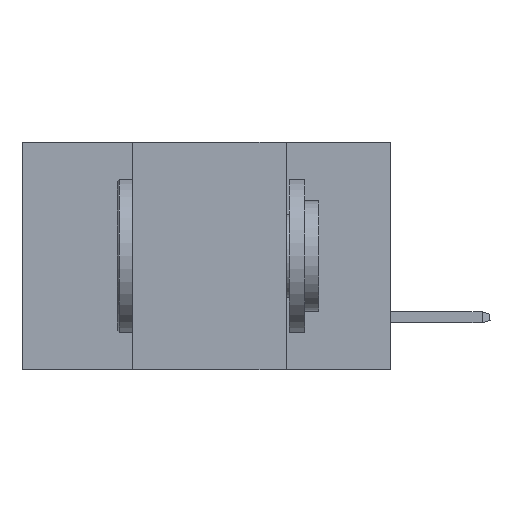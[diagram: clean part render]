
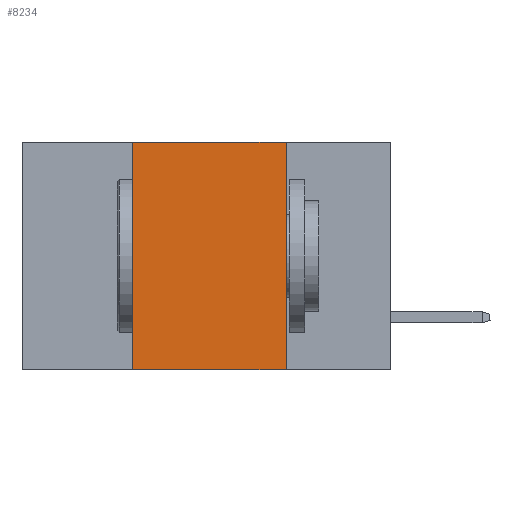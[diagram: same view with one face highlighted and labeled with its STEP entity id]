
A CAD part, left-side view. The second image highlights one B-rep face of the part: STEP entity #8234.
In plain terms, the highlighted planar face has unit normal (-1, 0, 0).
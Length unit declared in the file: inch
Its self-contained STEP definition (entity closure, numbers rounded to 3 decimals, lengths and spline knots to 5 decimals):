
#2219 = CARTESIAN_POINT ( 'NONE',  ( 0., 0.42, 0. ) ) ;
#3215 = ORIENTED_EDGE ( 'NONE', *, *, #3407, .F. ) ;
#3407 = EDGE_CURVE ( 'NONE', #5116, #25669, #23137, .T. ) ;
#4505 = EDGE_CURVE ( 'NONE', #23693, #37012, #13650, .T. ) ;
#5116 = VERTEX_POINT ( 'NONE', #27432 ) ;
#6448 = CARTESIAN_POINT ( 'NONE',  ( 0., 0.6, -0.37 ) ) ;
#6779 = ORIENTED_EDGE ( 'NONE', *, *, #24266, .T. ) ;
#7592 = DIRECTION ( 'NONE',  ( 1., 0., 0. ) ) ;
#7825 = CARTESIAN_POINT ( 'NONE',  ( 0., 0.17, -0.37 ) ) ;
#8042 = PLANE ( 'NONE',  #9699 ) ;
#8234 = ADVANCED_FACE ( 'NONE', ( #42196 ), #8042, .F. ) ;
#9063 = EDGE_CURVE ( 'NONE', #25669, #23693, #17835, .T. ) ;
#9699 = AXIS2_PLACEMENT_3D ( 'NONE', #18492, #7592, #40775 ) ;
#9901 = DIRECTION ( 'NONE',  ( 0., 0., 1. ) ) ;
#10714 = LINE ( 'NONE', #6448, #19375 ) ;
#13650 = LINE ( 'NONE', #19482, #45443 ) ;
#16788 = EDGE_LOOP ( 'NONE', ( #20616, #20183, #3215, #6779 ) ) ;
#17835 = LINE ( 'NONE', #19943, #41519 ) ;
#18492 = CARTESIAN_POINT ( 'NONE',  ( 0., 0.6, 0. ) ) ;
#19375 = VECTOR ( 'NONE', #32010, 39.37008 ) ;
#19482 = CARTESIAN_POINT ( 'NONE',  ( 0., 0.17, 0. ) ) ;
#19943 = CARTESIAN_POINT ( 'NONE',  ( 0., 0.6, 0. ) ) ;
#20183 = ORIENTED_EDGE ( 'NONE', *, *, #9063, .F. ) ;
#20616 = ORIENTED_EDGE ( 'NONE', *, *, #4505, .F. ) ;
#23137 = LINE ( 'NONE', #46650, #38188 ) ;
#23693 = VERTEX_POINT ( 'NONE', #35203 ) ;
#24266 = EDGE_CURVE ( 'NONE', #5116, #37012, #10714, .T. ) ;
#25669 = VERTEX_POINT ( 'NONE', #2219 ) ;
#27432 = CARTESIAN_POINT ( 'NONE',  ( 0., 0.42, -0.37 ) ) ;
#32010 = DIRECTION ( 'NONE',  ( 0., -1., 0. ) ) ;
#35203 = CARTESIAN_POINT ( 'NONE',  ( 0., 0.17, 0. ) ) ;
#37012 = VERTEX_POINT ( 'NONE', #7825 ) ;
#38188 = VECTOR ( 'NONE', #9901, 39.37008 ) ;
#38899 = DIRECTION ( 'NONE',  ( 0., -1., 0. ) ) ;
#40775 = DIRECTION ( 'NONE',  ( 0., 0., -1. ) ) ;
#41519 = VECTOR ( 'NONE', #38899, 39.37008 ) ;
#42196 = FACE_OUTER_BOUND ( 'NONE', #16788, .T. ) ;
#45373 = DIRECTION ( 'NONE',  ( 0., 0., -1. ) ) ;
#45443 = VECTOR ( 'NONE', #45373, 39.37008 ) ;
#46650 = CARTESIAN_POINT ( 'NONE',  ( 0., 0.42, 0. ) ) ;
